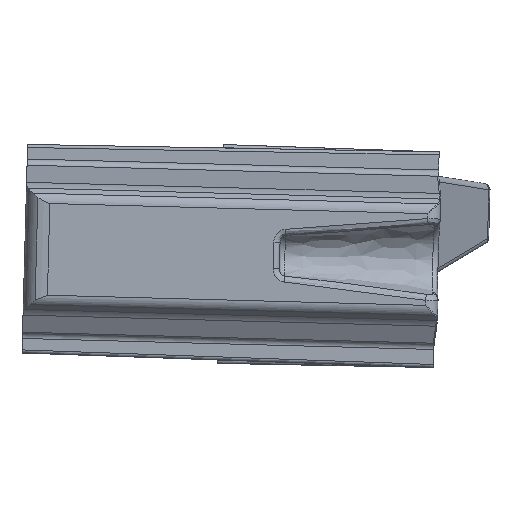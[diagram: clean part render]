
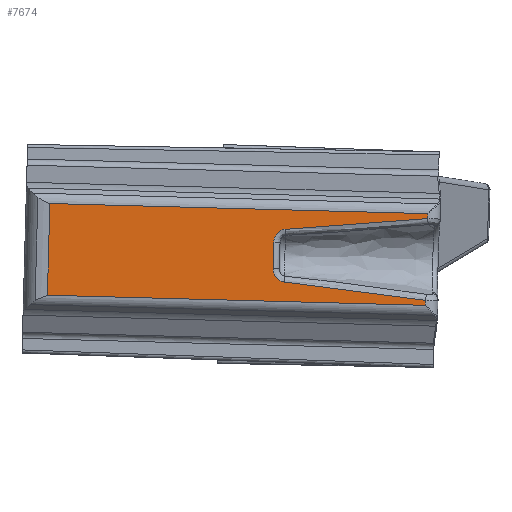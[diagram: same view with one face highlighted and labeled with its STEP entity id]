
A CAD part, front view. The second image highlights one B-rep face of the part: STEP entity #7674.
In plain terms, the highlighted face is planar.
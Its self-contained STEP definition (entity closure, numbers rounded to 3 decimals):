
#53 = AXIS2_PLACEMENT_3D ( 'NONE', #3073, #4262, #3666 ) ;
#123 = CARTESIAN_POINT ( 'NONE',  ( -28.946, -2.116, 20.868 ) ) ;
#151 = LINE ( 'NONE', #624, #7688 ) ;
#190 = EDGE_LOOP ( 'NONE', ( #1276, #317, #2804, #6098, #7522, #4840, #264, #3344, #7921, #1687 ) ) ;
#264 = ORIENTED_EDGE ( 'NONE', *, *, #1075, .F. ) ;
#317 = ORIENTED_EDGE ( 'NONE', *, *, #8018, .T. ) ;
#369 = CARTESIAN_POINT ( 'NONE',  ( -28.946, 2.474, 24.664 ) ) ;
#372 = EDGE_CURVE ( 'NONE', #7064, #5729, #2349, .T. ) ;
#386 = VECTOR ( 'NONE', #6778, 1000. ) ;
#516 = FACE_OUTER_BOUND ( 'NONE', #190, .T. ) ;
#584 = EDGE_CURVE ( 'NONE', #2880, #1713, #7798, .T. ) ;
#624 = CARTESIAN_POINT ( 'NONE',  ( -28.946, 6.7, 1.911 ) ) ;
#727 = CARTESIAN_POINT ( 'NONE',  ( -28.946, 2.066, 20.614 ) ) ;
#852 = B_SPLINE_CURVE_WITH_KNOTS ( 'NONE', 3,
 ( #5077, #7662, #727, #1973, #8246, #6466, #2575, #7741, #3837, #6956 ),
 .UNSPECIFIED., .F., .F.,
 ( 4, 2, 2, 2, 4 ),
 ( 0., 0., 0.001, 0.001, 0.002 ),
 .UNSPECIFIED. ) ;
#923 = EDGE_CURVE ( 'NONE', #4388, #3583, #3694, .T. ) ;
#995 = CARTESIAN_POINT ( 'NONE',  ( -28.946, 1.649, 19.954 ) ) ;
#1075 = EDGE_CURVE ( 'NONE', #1752, #5729, #852, .T. ) ;
#1168 = CARTESIAN_POINT ( 'NONE',  ( -28.946, -2.474, 24.664 ) ) ;
#1276 = ORIENTED_EDGE ( 'NONE', *, *, #5273, .T. ) ;
#1298 = LINE ( 'NONE', #4552, #4069 ) ;
#1353 = CARTESIAN_POINT ( 'NONE',  ( -28.946, 2.116, 20.868 ) ) ;
#1513 = CARTESIAN_POINT ( 'NONE',  ( -28.946, 3.281, 32.245 ) ) ;
#1634 = VECTOR ( 'NONE', #4228, 1000. ) ;
#1660 = CARTESIAN_POINT ( 'NONE',  ( -28.946, -2.104, 20.739 ) ) ;
#1687 = ORIENTED_EDGE ( 'NONE', *, *, #5874, .T. ) ;
#1713 = VERTEX_POINT ( 'NONE', #1513 ) ;
#1752 = VERTEX_POINT ( 'NONE', #1353 ) ;
#1973 = CARTESIAN_POINT ( 'NONE',  ( -28.946, 1.943, 20.385 ) ) ;
#2016 = DIRECTION ( 'NONE',  ( 0., 0., 1. ) ) ;
#2296 = CARTESIAN_POINT ( 'NONE',  ( -28.946, -1.304, 19.974 ) ) ;
#2297 = CARTESIAN_POINT ( 'NONE',  ( -28.946, 2.562, 25.613 ) ) ;
#2349 = LINE ( 'NONE', #995, #386 ) ;
#2407 = LINE ( 'NONE', #7696, #1634 ) ;
#2426 = CARTESIAN_POINT ( 'NONE',  ( -28.946, 2.207, 21.817 ) ) ;
#2436 = CARTESIAN_POINT ( 'NONE',  ( -28.946, -3.281, 32.245 ) ) ;
#2481 = EDGE_CURVE ( 'NONE', #1752, #1713, #5701, .T. ) ;
#2484 = CARTESIAN_POINT ( 'NONE',  ( -28.946, -2.562, 25.613 ) ) ;
#2539 = VECTOR ( 'NONE', #8308, 1000. ) ;
#2554 = DIRECTION ( 'NONE',  ( 0., -1., 0. ) ) ;
#2575 = CARTESIAN_POINT ( 'NONE',  ( -28.946, 1.548, 20.057 ) ) ;
#2804 = ORIENTED_EDGE ( 'NONE', *, *, #923, .F. ) ;
#2834 = VERTEX_POINT ( 'NONE', #4521 ) ;
#2880 = VERTEX_POINT ( 'NONE', #5485 ) ;
#2920 = CARTESIAN_POINT ( 'NONE',  ( -28.946, -3.679, 32.245 ) ) ;
#2972 = CARTESIAN_POINT ( 'NONE',  ( -28.946, 3.281, 32.245 ) ) ;
#2987 = EDGE_CURVE ( 'NONE', #4388, #3688, #3764, .T. ) ;
#3073 = CARTESIAN_POINT ( 'NONE',  ( -28.946, 6.7, 32.245 ) ) ;
#3110 = CARTESIAN_POINT ( 'NONE',  ( -28.946, -2.116, 20.868 ) ) ;
#3312 = CARTESIAN_POINT ( 'NONE',  ( -28.946, -3.679, 1.911 ) ) ;
#3324 = CARTESIAN_POINT ( 'NONE',  ( -28.946, -2.066, 20.614 ) ) ;
#3342 = VERTEX_POINT ( 'NONE', #3312 ) ;
#3344 = ORIENTED_EDGE ( 'NONE', *, *, #2481, .T. ) ;
#3583 = VERTEX_POINT ( 'NONE', #2920 ) ;
#3606 = VECTOR ( 'NONE', #7759, 1000. ) ;
#3666 = DIRECTION ( 'NONE',  ( 0., 0., -1. ) ) ;
#3688 = VERTEX_POINT ( 'NONE', #4562 ) ;
#3694 = LINE ( 'NONE', #6979, #2539 ) ;
#3700 = CARTESIAN_POINT ( 'NONE',  ( -28.946, -2.43, 24.189 ) ) ;
#3764 = B_SPLINE_CURVE_WITH_KNOTS ( 'NONE', 3,
 ( #2436, #7570, #4420, #6208, #2484, #1168, #3700, #4939, #7610, #3110 ),
 .UNSPECIFIED., .F., .F.,
 ( 4, 2, 2, 2, 4 ),
 ( 0., 0.006, 0.007, 0.009, 0.011 ),
 .UNSPECIFIED. ) ;
#3837 = CARTESIAN_POINT ( 'NONE',  ( -28.946, 1.175, 19.954 ) ) ;
#4069 = VECTOR ( 'NONE', #2016, 1000. ) ;
#4228 = DIRECTION ( 'NONE',  ( 0., 0., -1. ) ) ;
#4262 = DIRECTION ( 'NONE',  ( 1., 0., 0. ) ) ;
#4324 = CARTESIAN_POINT ( 'NONE',  ( -28.946, 2.43, 24.189 ) ) ;
#4388 = VERTEX_POINT ( 'NONE', #6531 ) ;
#4420 = CARTESIAN_POINT ( 'NONE',  ( -28.946, -2.859, 28.456 ) ) ;
#4521 = CARTESIAN_POINT ( 'NONE',  ( -28.946, 3.679, 1.911 ) ) ;
#4530 = CARTESIAN_POINT ( 'NONE',  ( -28.946, 6.7, 32.245 ) ) ;
#4552 = CARTESIAN_POINT ( 'NONE',  ( -28.946, -3.679, 32.245 ) ) ;
#4562 = CARTESIAN_POINT ( 'NONE',  ( -28.946, -2.116, 20.868 ) ) ;
#4589 = CARTESIAN_POINT ( 'NONE',  ( -28.946, -1.044, 19.954 ) ) ;
#4633 = CARTESIAN_POINT ( 'NONE',  ( -28.946, -1.662, 20.121 ) ) ;
#4719 = CARTESIAN_POINT ( 'NONE',  ( -28.946, -1.044, 19.954 ) ) ;
#4840 = ORIENTED_EDGE ( 'NONE', *, *, #372, .T. ) ;
#4885 = CARTESIAN_POINT ( 'NONE',  ( -28.946, -1.174, 19.954 ) ) ;
#4939 = CARTESIAN_POINT ( 'NONE',  ( -28.946, -2.297, 22.766 ) ) ;
#5077 = CARTESIAN_POINT ( 'NONE',  ( -28.946, 2.116, 20.868 ) ) ;
#5273 = EDGE_CURVE ( 'NONE', #2834, #3342, #151, .T. ) ;
#5485 = CARTESIAN_POINT ( 'NONE',  ( -28.946, 3.679, 32.245 ) ) ;
#5515 = CARTESIAN_POINT ( 'NONE',  ( -28.946, -1.86, 20.285 ) ) ;
#5561 = CARTESIAN_POINT ( 'NONE',  ( -28.946, 2.297, 22.766 ) ) ;
#5701 = B_SPLINE_CURVE_WITH_KNOTS ( 'NONE', 3,
 ( #6159, #2426, #5561, #4324, #369, #2297, #6894, #7436, #8183, #2972 ),
 .UNSPECIFIED., .F., .F.,
 ( 4, 2, 2, 2, 4 ),
 ( 0., 0.003, 0.004, 0.006, 0.011 ),
 .UNSPECIFIED. ) ;
#5729 = VERTEX_POINT ( 'NONE', #8002 ) ;
#5874 = EDGE_CURVE ( 'NONE', #2880, #2834, #2407, .T. ) ;
#6098 = ORIENTED_EDGE ( 'NONE', *, *, #2987, .T. ) ;
#6159 = CARTESIAN_POINT ( 'NONE',  ( -28.946, 2.116, 20.868 ) ) ;
#6208 = CARTESIAN_POINT ( 'NONE',  ( -28.946, -2.611, 26.087 ) ) ;
#6466 = CARTESIAN_POINT ( 'NONE',  ( -28.946, 1.66, 20.119 ) ) ;
#6531 = CARTESIAN_POINT ( 'NONE',  ( -28.946, -3.281, 32.245 ) ) ;
#6662 = CARTESIAN_POINT ( 'NONE',  ( -28.946, -1.547, 20.057 ) ) ;
#6778 = DIRECTION ( 'NONE',  ( 0., 1., 0. ) ) ;
#6894 = CARTESIAN_POINT ( 'NONE',  ( -28.946, 2.611, 26.087 ) ) ;
#6956 = CARTESIAN_POINT ( 'NONE',  ( -28.946, 1.044, 19.954 ) ) ;
#6979 = CARTESIAN_POINT ( 'NONE',  ( -28.946, 6.7, 32.245 ) ) ;
#7064 = VERTEX_POINT ( 'NONE', #4589 ) ;
#7110 = B_SPLINE_CURVE_WITH_KNOTS ( 'NONE', 3,
 ( #4719, #4885, #2296, #6662, #4633, #5515, #7435, #3324, #1660, #123 ),
 .UNSPECIFIED., .F., .F.,
 ( 4, 2, 2, 2, 4 ),
 ( 0., 0., 0.001, 0.001, 0.002 ),
 .UNSPECIFIED. ) ;
#7199 = EDGE_CURVE ( 'NONE', #7064, #3688, #7110, .T. ) ;
#7435 = CARTESIAN_POINT ( 'NONE',  ( -28.946, -1.944, 20.387 ) ) ;
#7436 = CARTESIAN_POINT ( 'NONE',  ( -28.946, 2.859, 28.456 ) ) ;
#7454 = PLANE ( 'NONE',  #53 ) ;
#7522 = ORIENTED_EDGE ( 'NONE', *, *, #7199, .F. ) ;
#7570 = CARTESIAN_POINT ( 'NONE',  ( -28.946, -3.07, 30.351 ) ) ;
#7610 = CARTESIAN_POINT ( 'NONE',  ( -28.946, -2.207, 21.817 ) ) ;
#7662 = CARTESIAN_POINT ( 'NONE',  ( -28.946, 2.104, 20.738 ) ) ;
#7674 = ADVANCED_FACE ( 'NONE', ( #516 ), #7454, .F. ) ;
#7688 = VECTOR ( 'NONE', #2554, 1000. ) ;
#7696 = CARTESIAN_POINT ( 'NONE',  ( -28.946, 3.679, 32.245 ) ) ;
#7741 = CARTESIAN_POINT ( 'NONE',  ( -28.946, 1.301, 19.973 ) ) ;
#7759 = DIRECTION ( 'NONE',  ( 0., -1., 0. ) ) ;
#7798 = LINE ( 'NONE', #4530, #3606 ) ;
#7921 = ORIENTED_EDGE ( 'NONE', *, *, #584, .F. ) ;
#8002 = CARTESIAN_POINT ( 'NONE',  ( -28.946, 1.044, 19.954 ) ) ;
#8018 = EDGE_CURVE ( 'NONE', #3342, #3583, #1298, .T. ) ;
#8183 = CARTESIAN_POINT ( 'NONE',  ( -28.946, 3.07, 30.351 ) ) ;
#8246 = CARTESIAN_POINT ( 'NONE',  ( -28.946, 1.86, 20.285 ) ) ;
#8308 = DIRECTION ( 'NONE',  ( 0., -1., 0. ) ) ;
